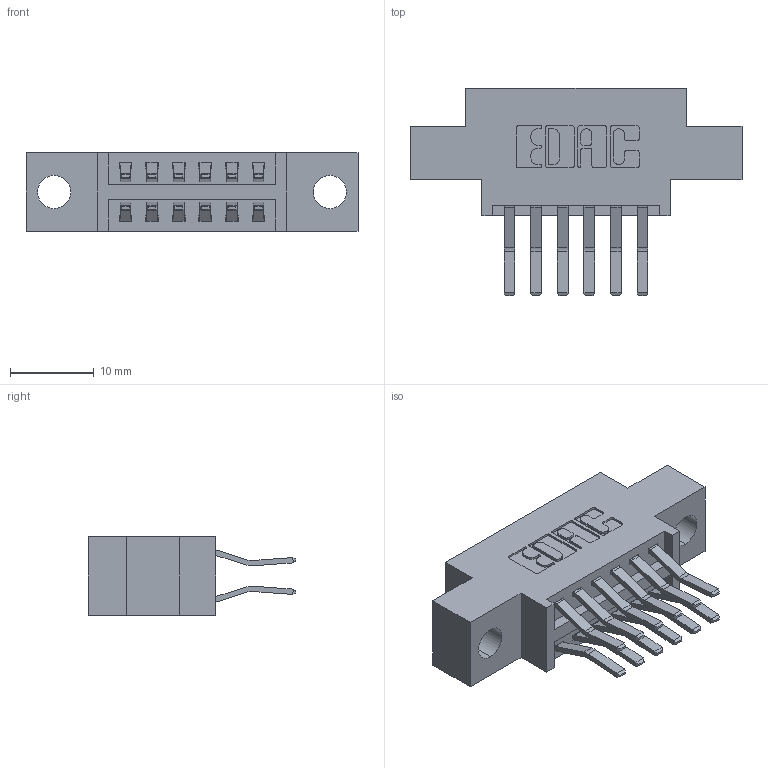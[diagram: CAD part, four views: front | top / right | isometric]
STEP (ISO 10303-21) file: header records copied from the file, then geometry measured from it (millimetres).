
FILE_DESCRIPTION (( 'STEP AP203' ), '1' );
FILE_NAME ('346-012-560-804.STEP', '2022-05-18T13:45:27', ( '' ), ( '' ), 'SwSTEP 2.0', 'SolidWorks 2020', '' );
FILE_SCHEMA (( 'CONFIG_CONTROL_DESIGN' ));
Length unit declared in the file: inch
Products named in the file (3): 346-012-560-804; 346 Part_0.170 Offset - 0.156 Dia-TH; 345-292-001_560 Tail
Assembly tree (13 placements, depth 2):
  346-012-560-804
    346 Part_0.170 Offset - 0.156 Dia-TH
    345-292-001_560 Tail  x12
Bounding box: 39.62 x 24.78 x 9.4 mm (x, y, z)
Volume: 3402.3 mm3; surface area: 4348.2 mm2
Topology: 13 solids, 13 shells, 788 faces, 2309 edges, 1522 vertices
Faces by surface type: plane 514, cylinder 274
Entity records: 9401 total; most frequent: CARTESIAN_POINT 1606, ORIENTED_EDGE 1538, DIRECTION 1469, EDGE_CURVE 769, VECTOR 609, LINE 609, VERTEX_POINT 510, AXIS2_PLACEMENT_3D 430
